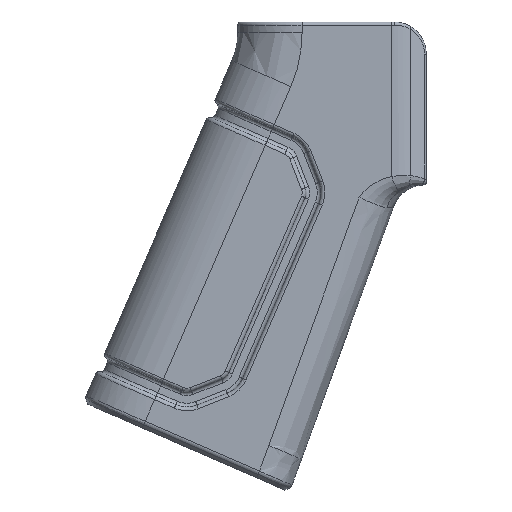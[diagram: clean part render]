
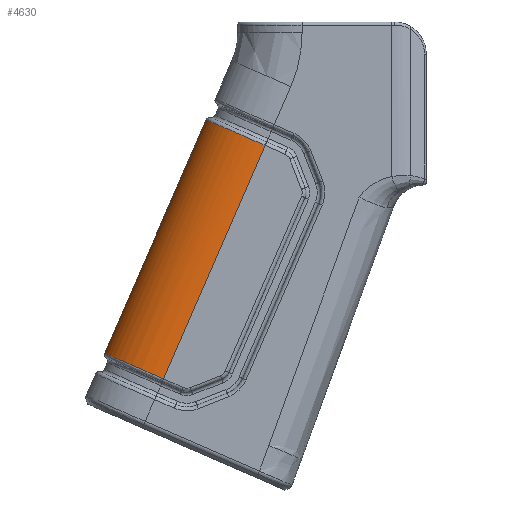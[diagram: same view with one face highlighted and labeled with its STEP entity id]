
A CAD part, left-side view. The second image highlights one B-rep face of the part: STEP entity #4630.
In plain terms, the highlighted free-form (B-spline) face has degree [2, 1] with [3, 2] control points.
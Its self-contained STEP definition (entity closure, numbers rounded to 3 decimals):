
#26=(
BOUNDED_SURFACE()
B_SPLINE_SURFACE(2,1,((#10943,#10944),(#10945,#10946),(#10947,#10948)),
 .UNSPECIFIED.,.F.,.F.,.F.)
B_SPLINE_SURFACE_WITH_KNOTS((3,3),(2,2),(-1.571,0.),
(0.,8.335),.UNSPECIFIED.)
GEOMETRIC_REPRESENTATION_ITEM()
RATIONAL_B_SPLINE_SURFACE(((1.,1.),(0.707,0.707),
(1.,1.)))
REPRESENTATION_ITEM('')
SURFACE()
);
#283=B_SPLINE_CURVE_WITH_KNOTS('',3,(#10662,#10663,#10664,#10665,#10666,
#10667,#10668,#10669,#10670,#10671,#10672,#10673),.UNSPECIFIED.,.F.,.F.,
(4,2,2,2,2,4),(0.,0.354,0.736,
1.169,1.46,1.738),.UNSPECIFIED.);
#294=B_SPLINE_CURVE_WITH_KNOTS('',3,(#10920,#10921,#10922,#10923,#10924,
#10925,#10926,#10927,#10928,#10929,#10930,#10931),.UNSPECIFIED.,.F.,.F.,
(4,2,2,2,2,4),(0.,0.276,0.568,1.002,
1.386,1.74),.UNSPECIFIED.);
#563=LINE('',#10940,#828);
#564=LINE('',#10942,#829);
#828=VECTOR('',#5848,10.);
#829=VECTOR('',#5851,10.);
#1201=FACE_OUTER_BOUND('',#1507,.T.);
#1507=EDGE_LOOP('',(#3723,#3724,#3725,#3726));
#2129=VERTEX_POINT('',#10659);
#2130=VERTEX_POINT('',#10661);
#2148=VERTEX_POINT('',#10840);
#2150=VERTEX_POINT('',#10905);
#2681=EDGE_CURVE('',#2129,#2130,#283,.T.);
#2715=EDGE_CURVE('',#2148,#2150,#294,.T.);
#2720=EDGE_CURVE('',#2148,#2130,#563,.T.);
#2721=EDGE_CURVE('',#2150,#2129,#564,.T.);
#3723=ORIENTED_EDGE('',*,*,#2715,.F.);
#3724=ORIENTED_EDGE('',*,*,#2720,.T.);
#3725=ORIENTED_EDGE('',*,*,#2681,.F.);
#3726=ORIENTED_EDGE('',*,*,#2721,.F.);
#4630=ADVANCED_FACE('',(#1201),#26,.T.);
#5848=DIRECTION('',(0.,-0.399,0.917));
#5851=DIRECTION('',(0.,-0.399,0.917));
#10659=CARTESIAN_POINT('',(-0.49,-110.866,-28.512));
#10661=CARTESIAN_POINT('',(-11.49,-122.503,-33.577));
#10662=CARTESIAN_POINT('Ctrl Pts',(-0.49,-110.866,
-28.512));
#10663=CARTESIAN_POINT('Ctrl Pts',(-1.769,-110.866,
-28.512));
#10664=CARTESIAN_POINT('Ctrl Pts',(-3.056,-111.108,
-28.618));
#10665=CARTESIAN_POINT('Ctrl Pts',(-5.512,-112.051,-29.028));
#10666=CARTESIAN_POINT('Ctrl Pts',(-6.677,-112.786,
-29.348));
#10667=CARTESIAN_POINT('Ctrl Pts',(-8.744,-114.661,-30.164));
#10668=CARTESIAN_POINT('Ctrl Pts',(-9.617,-115.849,
-30.681));
#10669=CARTESIAN_POINT('Ctrl Pts',(-10.672,-117.994,
-31.615));
#10670=CARTESIAN_POINT('Ctrl Pts',(-10.99,-118.905,
-32.011));
#10671=CARTESIAN_POINT('Ctrl Pts',(-11.393,-120.713,-32.799));
#10672=CARTESIAN_POINT('Ctrl Pts',(-11.49,-121.608,
-33.188));
#10673=CARTESIAN_POINT('Ctrl Pts',(-11.49,-122.503,-33.577));
#10840=CARTESIAN_POINT('',(-11.49,-102.454,-79.635));
#10905=CARTESIAN_POINT('',(-0.49,-90.817,-74.569));
#10920=CARTESIAN_POINT('Ctrl Pts',(-11.49,-102.454,
-79.635));
#10921=CARTESIAN_POINT('Ctrl Pts',(-11.49,-101.564,
-79.247));
#10922=CARTESIAN_POINT('Ctrl Pts',(-11.393,-100.664,
-78.855));
#10923=CARTESIAN_POINT('Ctrl Pts',(-10.988,-98.851,
-78.066));
#10924=CARTESIAN_POINT('Ctrl Pts',(-10.672,-97.944,
-77.672));
#10925=CARTESIAN_POINT('Ctrl Pts',(-9.618,-95.802,
-76.739));
#10926=CARTESIAN_POINT('Ctrl Pts',(-8.744,-94.611,
-76.221));
#10927=CARTESIAN_POINT('Ctrl Pts',(-6.67,-92.732,
-75.403));
#10928=CARTESIAN_POINT('Ctrl Pts',(-5.512,-92.002,
-75.085));
#10929=CARTESIAN_POINT('Ctrl Pts',(-3.056,-91.061,-74.676));
#10930=CARTESIAN_POINT('Ctrl Pts',(-1.771,-90.817,-74.569));
#10931=CARTESIAN_POINT('Ctrl Pts',(-0.49,-90.817,
-74.569));
#10940=CARTESIAN_POINT('',(-11.49,-127.561,-21.956));
#10942=CARTESIAN_POINT('',(-0.49,-115.924,-16.89));
#10943=CARTESIAN_POINT('Ctrl Pts',(-11.49,-127.561,
-21.956));
#10944=CARTESIAN_POINT('Ctrl Pts',(-11.49,-94.295,
-98.38));
#10945=CARTESIAN_POINT('Ctrl Pts',(-11.49,-115.924,-16.89));
#10946=CARTESIAN_POINT('Ctrl Pts',(-11.49,-82.658,
-93.314));
#10947=CARTESIAN_POINT('Ctrl Pts',(-0.49,-115.924,-16.89));
#10948=CARTESIAN_POINT('Ctrl Pts',(-0.49,-82.658,
-93.314));
